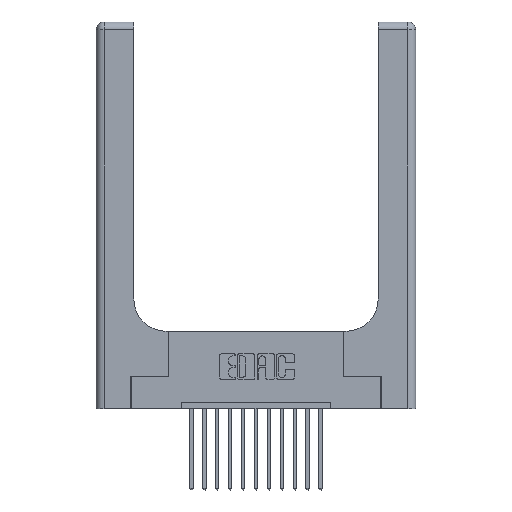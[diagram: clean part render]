
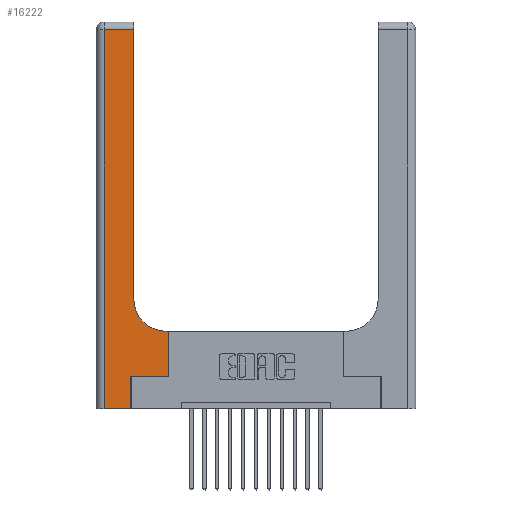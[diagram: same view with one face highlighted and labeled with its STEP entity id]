
A CAD part, top view. The second image highlights one B-rep face of the part: STEP entity #16222.
In plain terms, the highlighted planar face has unit normal (0, 0, 1).
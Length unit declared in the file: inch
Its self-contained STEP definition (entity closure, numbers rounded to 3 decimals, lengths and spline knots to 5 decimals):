
#459 = CARTESIAN_POINT ( 'NONE',  ( 0.269, 0., 0.37 ) ) ;
#593 = CARTESIAN_POINT ( 'NONE',  ( 0., 2.94, 0.37 ) ) ;
#1093 = CARTESIAN_POINT ( 'NONE',  ( 0.06, 3., 0.37 ) ) ;
#1210 = LINE ( 'NONE', #459, #9974 ) ;
#1738 = ORIENTED_EDGE ( 'NONE', *, *, #1973, .T. ) ;
#1847 = VECTOR ( 'NONE', #10872, 39.37008 ) ;
#1865 = CARTESIAN_POINT ( 'NONE',  ( 0.269, 0., 0.37 ) ) ;
#1973 = EDGE_CURVE ( 'NONE', #8148, #11749, #12412, .T. ) ;
#2156 = CARTESIAN_POINT ( 'NONE',  ( 0.269, 0.25, 0.37 ) ) ;
#2277 = CARTESIAN_POINT ( 'NONE',  ( 0.5585, 0.6, 0.37 ) ) ;
#2490 = LINE ( 'NONE', #2156, #1847 ) ;
#2607 = CARTESIAN_POINT ( 'NONE',  ( 0.06, 0., 0.37 ) ) ;
#2714 = CARTESIAN_POINT ( 'NONE',  ( 0.269, 0.25, 0.37 ) ) ;
#2759 = CARTESIAN_POINT ( 'NONE',  ( 0.5585, 0.25, 0.37 ) ) ;
#3105 = CIRCLE ( 'NONE', #12607, 0.25 ) ;
#3164 = ORIENTED_EDGE ( 'NONE', *, *, #4520, .T. ) ;
#3356 = DIRECTION ( 'NONE',  ( 0., 1., 0. ) ) ;
#4369 = LINE ( 'NONE', #12177, #16371 ) ;
#4520 = EDGE_CURVE ( 'NONE', #9150, #16577, #3105, .T. ) ;
#4699 = ORIENTED_EDGE ( 'NONE', *, *, #11893, .T. ) ;
#5375 = CARTESIAN_POINT ( 'NONE',  ( 0.5415, 0.6, 0.37 ) ) ;
#5549 = CARTESIAN_POINT ( 'NONE',  ( 0., 3., 0.37 ) ) ;
#5851 = VECTOR ( 'NONE', #6943, 39.37008 ) ;
#5886 = DIRECTION ( 'NONE',  ( -1., 0., 0. ) ) ;
#6346 = ORIENTED_EDGE ( 'NONE', *, *, #12724, .T. ) ;
#6565 = CARTESIAN_POINT ( 'NONE',  ( 0.2915, 0.85, 0.37 ) ) ;
#6736 = CARTESIAN_POINT ( 'NONE',  ( 0.5415, 0.85, 0.37 ) ) ;
#6912 = EDGE_LOOP ( 'NONE', ( #6346, #16720, #10749, #4699, #14450, #12180, #1738, #13162, #3164 ) ) ;
#6943 = DIRECTION ( 'NONE',  ( 0., -1., 0. ) ) ;
#7085 = VECTOR ( 'NONE', #10142, 39.37008 ) ;
#7780 = EDGE_CURVE ( 'NONE', #16049, #14737, #10702, .T. ) ;
#8083 = DIRECTION ( 'NONE',  ( 0., 0., -1. ) ) ;
#8109 = DIRECTION ( 'NONE',  ( 1., 0., 0. ) ) ;
#8148 = VERTEX_POINT ( 'NONE', #2759 ) ;
#8710 = VECTOR ( 'NONE', #5886, 39.37008 ) ;
#9115 = LINE ( 'NONE', #10354, #15086 ) ;
#9150 = VERTEX_POINT ( 'NONE', #5375 ) ;
#9256 = CARTESIAN_POINT ( 'NONE',  ( 0.06, 2.94, 0.37 ) ) ;
#9287 = CARTESIAN_POINT ( 'NONE',  ( 0.5585, 0.25, 0.37 ) ) ;
#9452 = PLANE ( 'NONE',  #16259 ) ;
#9974 = VECTOR ( 'NONE', #3356, 39.37008 ) ;
#10142 = DIRECTION ( 'NONE',  ( -1., 0., 0. ) ) ;
#10354 = CARTESIAN_POINT ( 'NONE',  ( 0.2915, 3., 0.37 ) ) ;
#10457 = CARTESIAN_POINT ( 'NONE',  ( 0.2915, 2.94, 0.37 ) ) ;
#10702 = LINE ( 'NONE', #593, #7085 ) ;
#10749 = ORIENTED_EDGE ( 'NONE', *, *, #16130, .T. ) ;
#10872 = DIRECTION ( 'NONE',  ( 1., 0., 0. ) ) ;
#11207 = EDGE_CURVE ( 'NONE', #15003, #8148, #2490, .T. ) ;
#11668 = EDGE_CURVE ( 'NONE', #12598, #15003, #1210, .T. ) ;
#11749 = VERTEX_POINT ( 'NONE', #2277 ) ;
#11893 = EDGE_CURVE ( 'NONE', #17170, #12598, #4369, .T. ) ;
#12046 = FACE_OUTER_BOUND ( 'NONE', #6912, .T. ) ;
#12177 = CARTESIAN_POINT ( 'NONE',  ( 0., 0., 0.37 ) ) ;
#12180 = ORIENTED_EDGE ( 'NONE', *, *, #11207, .T. ) ;
#12412 = LINE ( 'NONE', #9287, #13916 ) ;
#12598 = VERTEX_POINT ( 'NONE', #1865 ) ;
#12607 = AXIS2_PLACEMENT_3D ( 'NONE', #6736, #16276, #8109 ) ;
#12724 = EDGE_CURVE ( 'NONE', #16577, #16049, #9115, .T. ) ;
#13162 = ORIENTED_EDGE ( 'NONE', *, *, #15048, .T. ) ;
#13228 = DIRECTION ( 'NONE',  ( 0., 1., 0. ) ) ;
#13337 = DIRECTION ( 'NONE',  ( 1., 0., 0. ) ) ;
#13916 = VECTOR ( 'NONE', #13228, 39.37008 ) ;
#14450 = ORIENTED_EDGE ( 'NONE', *, *, #11668, .T. ) ;
#14737 = VERTEX_POINT ( 'NONE', #9256 ) ;
#15003 = VERTEX_POINT ( 'NONE', #2714 ) ;
#15048 = EDGE_CURVE ( 'NONE', #11749, #9150, #15317, .T. ) ;
#15086 = VECTOR ( 'NONE', #17207, 39.37008 ) ;
#15317 = LINE ( 'NONE', #15383, #8710 ) ;
#15383 = CARTESIAN_POINT ( 'NONE',  ( 0.2915, 0.6, 0.37 ) ) ;
#16049 = VERTEX_POINT ( 'NONE', #10457 ) ;
#16130 = EDGE_CURVE ( 'NONE', #14737, #17170, #16325, .T. ) ;
#16222 = ADVANCED_FACE ( 'NONE', ( #12046 ), #9452, .F. ) ;
#16259 = AXIS2_PLACEMENT_3D ( 'NONE', #5549, #8083, #16367 ) ;
#16276 = DIRECTION ( 'NONE',  ( 0., 0., -1. ) ) ;
#16325 = LINE ( 'NONE', #1093, #5851 ) ;
#16367 = DIRECTION ( 'NONE',  ( -1., 0., 0. ) ) ;
#16371 = VECTOR ( 'NONE', #13337, 39.37008 ) ;
#16577 = VERTEX_POINT ( 'NONE', #6565 ) ;
#16720 = ORIENTED_EDGE ( 'NONE', *, *, #7780, .T. ) ;
#17170 = VERTEX_POINT ( 'NONE', #2607 ) ;
#17207 = DIRECTION ( 'NONE',  ( 0., 1., 0. ) ) ;
